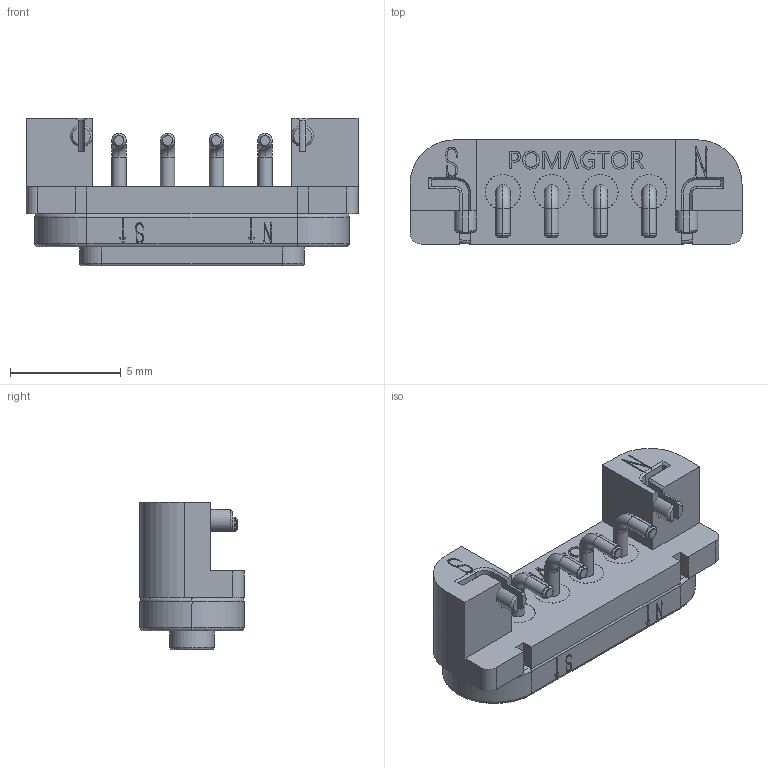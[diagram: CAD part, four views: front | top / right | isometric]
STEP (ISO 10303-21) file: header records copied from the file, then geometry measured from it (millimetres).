
FILE_DESCRIPTION (( 'STEP AP203' ), '1' );
FILE_NAME ('686-F0432350125.STEP', '2023-02-14T11:36:28', ( 'Magnum' ), ( '' ), 'SwSTEP 2.0', 'SolidWorks 2020', '' );
FILE_SCHEMA (( 'CONFIG_CONTROL_DESIGN' ));
Length unit declared in the file: millimetre
Products named in the file (1): 686-F0432350125
Bounding box: 15 x 4.7 x 6.66 mm (x, y, z)
Surface area: 956.1 mm2 (no closed solid volume)
Topology: 0 solids, 243 shells, 2912 faces, 6301 edges, 4162 vertices
Faces by surface type: plane 2076, cylinder 604, bspline 144, cone 54, torus 34
Entity records: 85793 total; most frequent: CARTESIAN_POINT 22503, ORIENTED_EDGE 12602, DIRECTION 12596, EDGE_CURVE 6301, LINE 4482, VECTOR 4482, VERTEX_POINT 4162, AXIS2_PLACEMENT_3D 4057
